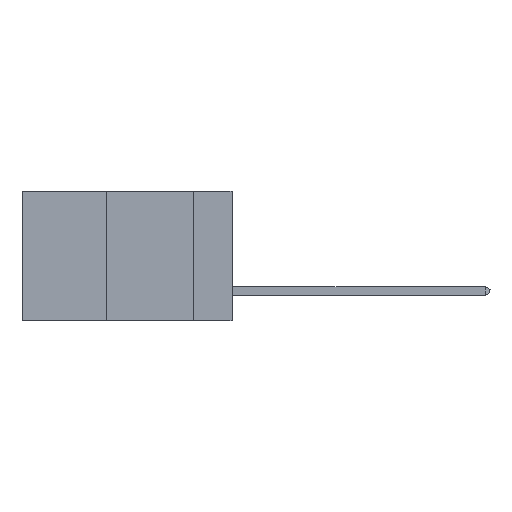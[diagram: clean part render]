
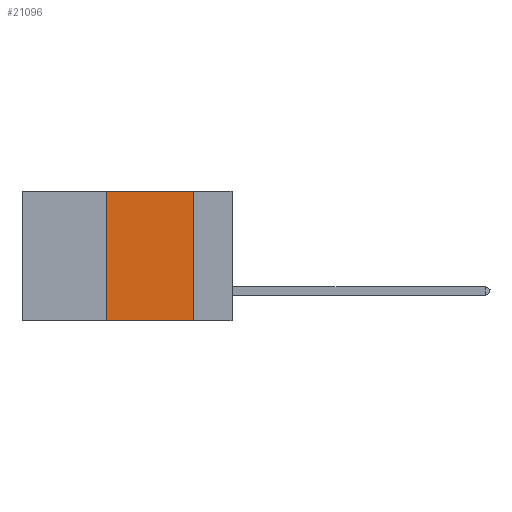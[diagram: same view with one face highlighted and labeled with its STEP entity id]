
A CAD part, left-side view. The second image highlights one B-rep face of the part: STEP entity #21096.
In plain terms, the highlighted planar face has unit normal (-1, 0, 0).
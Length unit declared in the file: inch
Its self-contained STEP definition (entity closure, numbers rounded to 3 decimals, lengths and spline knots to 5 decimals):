
#111 = CARTESIAN_POINT ( 'NONE',  ( 0., 0.36, 0. ) ) ;
#290 = CARTESIAN_POINT ( 'NONE',  ( 0., 0.36, -0.37 ) ) ;
#703 = EDGE_CURVE ( 'NONE', #9616, #4419, #16795, .T. ) ;
#2369 = CARTESIAN_POINT ( 'NONE',  ( 0., 0.11, -0.37 ) ) ;
#3182 = EDGE_LOOP ( 'NONE', ( #19954, #6479, #8183, #15478 ) ) ;
#3391 = VERTEX_POINT ( 'NONE', #11530 ) ;
#4055 = PLANE ( 'NONE',  #9739 ) ;
#4288 = CARTESIAN_POINT ( 'NONE',  ( 0., 0.6, -0.37 ) ) ;
#4419 = VERTEX_POINT ( 'NONE', #2369 ) ;
#4792 = DIRECTION ( 'NONE',  ( 0., -1., 0. ) ) ;
#5899 = VECTOR ( 'NONE', #4792, 39.37008 ) ;
#6479 = ORIENTED_EDGE ( 'NONE', *, *, #6822, .F. ) ;
#6822 = EDGE_CURVE ( 'NONE', #3391, #15957, #8772, .T. ) ;
#7325 = EDGE_CURVE ( 'NONE', #15957, #4419, #17132, .T. ) ;
#8183 = ORIENTED_EDGE ( 'NONE', *, *, #16989, .F. ) ;
#8517 = FACE_OUTER_BOUND ( 'NONE', #3182, .T. ) ;
#8772 = LINE ( 'NONE', #9765, #5899 ) ;
#9005 = LINE ( 'NONE', #111, #13966 ) ;
#9616 = VERTEX_POINT ( 'NONE', #290 ) ;
#9739 = AXIS2_PLACEMENT_3D ( 'NONE', #15891, #17425, #20786 ) ;
#9765 = CARTESIAN_POINT ( 'NONE',  ( 0., 0.6, 0. ) ) ;
#11134 = VECTOR ( 'NONE', #18819, 39.37008 ) ;
#11530 = CARTESIAN_POINT ( 'NONE',  ( 0., 0.36, 0. ) ) ;
#13966 = VECTOR ( 'NONE', #15126, 39.37008 ) ;
#15126 = DIRECTION ( 'NONE',  ( 0., 0., 1. ) ) ;
#15230 = VECTOR ( 'NONE', #19639, 39.37008 ) ;
#15478 = ORIENTED_EDGE ( 'NONE', *, *, #703, .T. ) ;
#15891 = CARTESIAN_POINT ( 'NONE',  ( 0., 0.6, 0. ) ) ;
#15957 = VERTEX_POINT ( 'NONE', #16631 ) ;
#16631 = CARTESIAN_POINT ( 'NONE',  ( 0., 0.11, 0. ) ) ;
#16795 = LINE ( 'NONE', #4288, #15230 ) ;
#16989 = EDGE_CURVE ( 'NONE', #9616, #3391, #9005, .T. ) ;
#17132 = LINE ( 'NONE', #20632, #11134 ) ;
#17425 = DIRECTION ( 'NONE',  ( 1., 0., 0. ) ) ;
#18819 = DIRECTION ( 'NONE',  ( 0., 0., -1. ) ) ;
#19639 = DIRECTION ( 'NONE',  ( 0., -1., 0. ) ) ;
#19954 = ORIENTED_EDGE ( 'NONE', *, *, #7325, .F. ) ;
#20632 = CARTESIAN_POINT ( 'NONE',  ( 0., 0.11, 0. ) ) ;
#20786 = DIRECTION ( 'NONE',  ( 0., 0., -1. ) ) ;
#21096 = ADVANCED_FACE ( 'NONE', ( #8517 ), #4055, .F. ) ;
